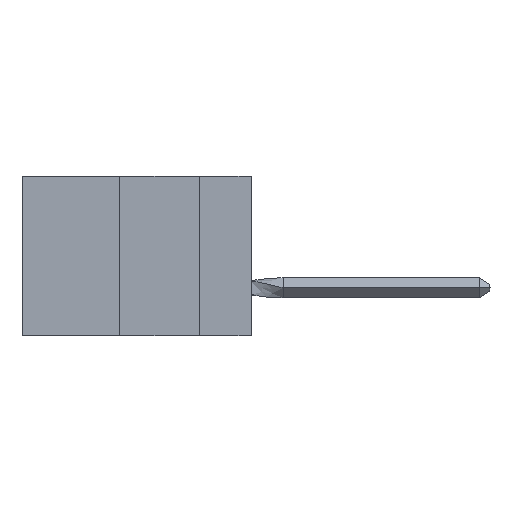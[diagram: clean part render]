
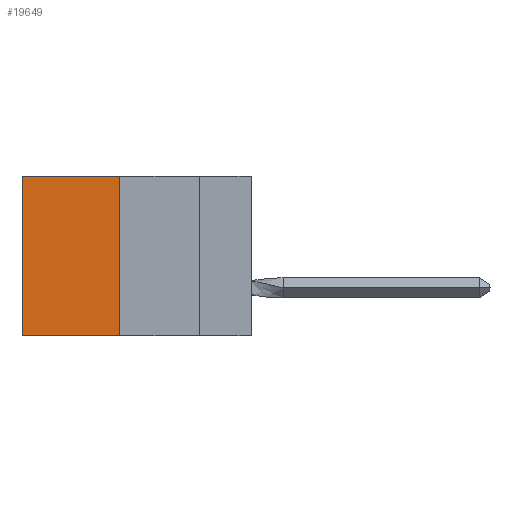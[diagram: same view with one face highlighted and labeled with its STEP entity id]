
A CAD part, left-side view. The second image highlights one B-rep face of the part: STEP entity #19649.
In plain terms, the highlighted planar face has unit normal (-1, 0, 0).
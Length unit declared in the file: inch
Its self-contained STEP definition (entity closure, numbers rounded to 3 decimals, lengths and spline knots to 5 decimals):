
#3597 = EDGE_CURVE ( 'NONE', #16464, #11294, #11771, .T. ) ;
#3836 = DIRECTION ( 'NONE',  ( 0., 0., -1. ) ) ;
#3968 = DIRECTION ( 'NONE',  ( 1., 0., 0. ) ) ;
#4132 = DIRECTION ( 'NONE',  ( 0., 1., 0. ) ) ;
#5067 = DIRECTION ( 'NONE',  ( 0., 0., -1. ) ) ;
#5926 = DIRECTION ( 'NONE',  ( 0., 0., -1. ) ) ;
#7660 = CARTESIAN_POINT ( 'NONE',  ( 0.305, 0.413, -0.5 ) ) ;
#8492 = LINE ( 'NONE', #11116, #11877 ) ;
#8618 = CARTESIAN_POINT ( 'NONE',  ( 0.305, 0.413, -0.5 ) ) ;
#8874 = EDGE_LOOP ( 'NONE', ( #16768, #9089, #16890, #13622 ) ) ;
#9089 = ORIENTED_EDGE ( 'NONE', *, *, #20027, .F. ) ;
#9143 = LINE ( 'NONE', #7660, #18380 ) ;
#9520 = FACE_OUTER_BOUND ( 'NONE', #8874, .T. ) ;
#9602 = VECTOR ( 'NONE', #16038, 39.37008 ) ;
#11116 = CARTESIAN_POINT ( 'NONE',  ( 0.305, 0.72, -0.5 ) ) ;
#11294 = VERTEX_POINT ( 'NONE', #13766 ) ;
#11462 = EDGE_CURVE ( 'NONE', #16464, #13337, #9143, .T. ) ;
#11771 = LINE ( 'NONE', #14493, #9602 ) ;
#11877 = VECTOR ( 'NONE', #5067, 39.37008 ) ;
#13070 = PLANE ( 'NONE',  #15409 ) ;
#13337 = VERTEX_POINT ( 'NONE', #15684 ) ;
#13521 = CARTESIAN_POINT ( 'NONE',  ( 0.305, 0.413, -0.5 ) ) ;
#13622 = ORIENTED_EDGE ( 'NONE', *, *, #3597, .T. ) ;
#13766 = CARTESIAN_POINT ( 'NONE',  ( 0.305, 0.72, 0. ) ) ;
#14493 = CARTESIAN_POINT ( 'NONE',  ( 0.305, 0.413, 0. ) ) ;
#14598 = LINE ( 'NONE', #13521, #17029 ) ;
#14727 = VERTEX_POINT ( 'NONE', #18243 ) ;
#15306 = EDGE_CURVE ( 'NONE', #11294, #14727, #8492, .T. ) ;
#15409 = AXIS2_PLACEMENT_3D ( 'NONE', #8618, #3968, #3836 ) ;
#15684 = CARTESIAN_POINT ( 'NONE',  ( 0.305, 0.413, -0.5 ) ) ;
#16038 = DIRECTION ( 'NONE',  ( 0., 1., 0. ) ) ;
#16464 = VERTEX_POINT ( 'NONE', #17844 ) ;
#16768 = ORIENTED_EDGE ( 'NONE', *, *, #15306, .T. ) ;
#16890 = ORIENTED_EDGE ( 'NONE', *, *, #11462, .F. ) ;
#17029 = VECTOR ( 'NONE', #4132, 39.37008 ) ;
#17844 = CARTESIAN_POINT ( 'NONE',  ( 0.305, 0.413, 0. ) ) ;
#18243 = CARTESIAN_POINT ( 'NONE',  ( 0.305, 0.72, -0.5 ) ) ;
#18380 = VECTOR ( 'NONE', #5926, 39.37008 ) ;
#19649 = ADVANCED_FACE ( 'NONE', ( #9520 ), #13070, .F. ) ;
#20027 = EDGE_CURVE ( 'NONE', #13337, #14727, #14598, .T. ) ;
